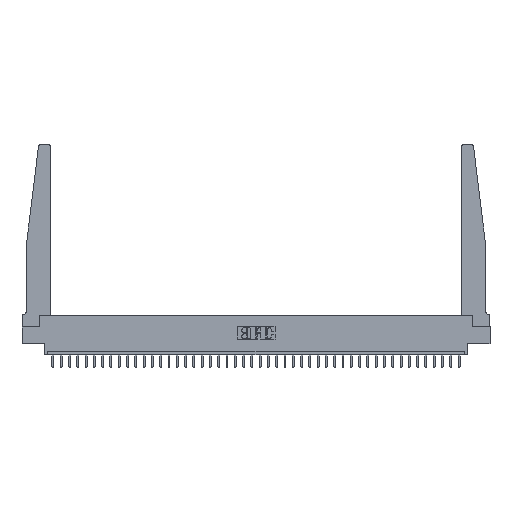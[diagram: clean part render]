
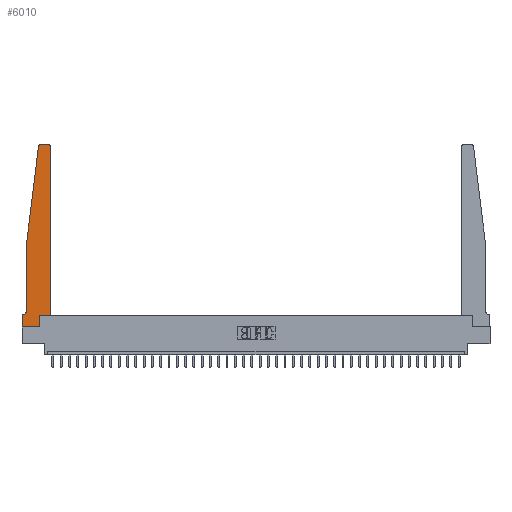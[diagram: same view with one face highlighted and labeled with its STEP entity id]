
A CAD part, top view. The second image highlights one B-rep face of the part: STEP entity #6010.
In plain terms, the highlighted planar face has unit normal (0, 0, 1).
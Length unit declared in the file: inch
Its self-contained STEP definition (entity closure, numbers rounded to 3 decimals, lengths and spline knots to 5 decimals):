
#558 = CARTESIAN_POINT ( 'NONE',  ( 0.065, 1.25, 0.37 ) ) ;
#587 = CARTESIAN_POINT ( 'NONE',  ( 0.065, 1.25, 0.37 ) ) ;
#779 = VECTOR ( 'NONE', #24021, 39.37008 ) ;
#856 = VERTEX_POINT ( 'NONE', #21070 ) ;
#1024 = VERTEX_POINT ( 'NONE', #10144 ) ;
#1655 = DIRECTION ( 'NONE',  ( 0., 1., 0. ) ) ;
#1832 = CARTESIAN_POINT ( 'NONE',  ( 0., 0.1875, 0.37 ) ) ;
#2166 = DIRECTION ( 'NONE',  ( 0., 0., -1. ) ) ;
#2306 = CARTESIAN_POINT ( 'NONE',  ( 0.27653, 2.72, 0.37 ) ) ;
#3428 = EDGE_CURVE ( 'NONE', #25080, #15302, #9215, .T. ) ;
#4819 = DIRECTION ( 'NONE',  ( 0., -1., 0. ) ) ;
#5062 = LINE ( 'NONE', #22486, #21195 ) ;
#5233 = VECTOR ( 'NONE', #21370, 39.37008 ) ;
#5399 = AXIS2_PLACEMENT_3D ( 'NONE', #24144, #2166, #29606 ) ;
#6010 = ADVANCED_FACE ( 'NONE', ( #11572 ), #15756, .T. ) ;
#6064 = EDGE_CURVE ( 'NONE', #11820, #20623, #17079, .T. ) ;
#6238 = LINE ( 'NONE', #587, #24451 ) ;
#6277 = EDGE_CURVE ( 'NONE', #20623, #12182, #6449, .T. ) ;
#6449 = CIRCLE ( 'NONE', #5399, 0.05 ) ;
#6466 = DIRECTION ( 'NONE',  ( 1., 0., 0. ) ) ;
#6562 = ORIENTED_EDGE ( 'NONE', *, *, #6064, .T. ) ;
#7493 = CARTESIAN_POINT ( 'NONE',  ( 0.425, 0.18, 0.37 ) ) ;
#9215 = LINE ( 'NONE', #16953, #24053 ) ;
#9612 = EDGE_CURVE ( 'NONE', #856, #20183, #13730, .T. ) ;
#9614 = CARTESIAN_POINT ( 'NONE',  ( 0.065, 0.1875, 0.37 ) ) ;
#9707 = LINE ( 'NONE', #13720, #34671 ) ;
#9741 = ORIENTED_EDGE ( 'NONE', *, *, #3428, .T. ) ;
#9880 = CARTESIAN_POINT ( 'NONE',  ( 0., 0., 0.37 ) ) ;
#10144 = CARTESIAN_POINT ( 'NONE',  ( 0., 0.1875, 0.37 ) ) ;
#10590 = AXIS2_PLACEMENT_3D ( 'NONE', #2306, #18377, #20989 ) ;
#11152 = LINE ( 'NONE', #9614, #17508 ) ;
#11572 = FACE_OUTER_BOUND ( 'NONE', #13483, .T. ) ;
#11820 = VERTEX_POINT ( 'NONE', #558 ) ;
#12182 = VERTEX_POINT ( 'NONE', #18285 ) ;
#12961 = CARTESIAN_POINT ( 'NONE',  ( 0.2605, 0.18, 0.37 ) ) ;
#13011 = EDGE_CURVE ( 'NONE', #1024, #16116, #9707, .T. ) ;
#13483 = EDGE_LOOP ( 'NONE', ( #28236, #22872, #15942, #6562, #14716, #17253, #27853, #21264, #21352, #15032, #9741, #23097 ) ) ;
#13720 = CARTESIAN_POINT ( 'NONE',  ( 0., 0., 0.37 ) ) ;
#13730 = LINE ( 'NONE', #12961, #5233 ) ;
#14716 = ORIENTED_EDGE ( 'NONE', *, *, #6277, .T. ) ;
#14963 = CARTESIAN_POINT ( 'NONE',  ( 0.27653, 2.75, 0.37 ) ) ;
#15032 = ORIENTED_EDGE ( 'NONE', *, *, #30413, .T. ) ;
#15148 = AXIS2_PLACEMENT_3D ( 'NONE', #1832, #18485, #32083 ) ;
#15302 = VERTEX_POINT ( 'NONE', #17391 ) ;
#15756 = PLANE ( 'NONE',  #15148 ) ;
#15942 = ORIENTED_EDGE ( 'NONE', *, *, #27890, .T. ) ;
#16116 = VERTEX_POINT ( 'NONE', #9880 ) ;
#16468 = DIRECTION ( 'NONE',  ( 0., -1., 0. ) ) ;
#16653 = EDGE_CURVE ( 'NONE', #24410, #29424, #30445, .T. ) ;
#16739 = AXIS2_PLACEMENT_3D ( 'NONE', #28509, #25639, #6466 ) ;
#16872 = DIRECTION ( 'NONE',  ( -0.122, -0.992, 0. ) ) ;
#16953 = CARTESIAN_POINT ( 'NONE',  ( 0.425, 0.18, 0.37 ) ) ;
#17079 = LINE ( 'NONE', #34515, #32295 ) ;
#17162 = CARTESIAN_POINT ( 'NONE',  ( 0.425, 0.18, 0.37 ) ) ;
#17253 = ORIENTED_EDGE ( 'NONE', *, *, #20396, .T. ) ;
#17391 = CARTESIAN_POINT ( 'NONE',  ( 0.425, 2.72, 0.37 ) ) ;
#17508 = VECTOR ( 'NONE', #18240, 39.37008 ) ;
#18240 = DIRECTION ( 'NONE',  ( -1., 0., 0. ) ) ;
#18285 = CARTESIAN_POINT ( 'NONE',  ( 0.015, 0.1875, 0.37 ) ) ;
#18377 = DIRECTION ( 'NONE',  ( 0., 0., 1. ) ) ;
#18485 = DIRECTION ( 'NONE',  ( 0., 0., 1. ) ) ;
#19468 = CARTESIAN_POINT ( 'NONE',  ( 0.2605, 0.18, 0.37 ) ) ;
#20010 = DIRECTION ( 'NONE',  ( -1., 0., 0. ) ) ;
#20183 = VERTEX_POINT ( 'NONE', #19468 ) ;
#20298 = CARTESIAN_POINT ( 'NONE',  ( 0.395, 2.75, 0.37 ) ) ;
#20396 = EDGE_CURVE ( 'NONE', #12182, #1024, #11152, .T. ) ;
#20623 = VERTEX_POINT ( 'NONE', #24862 ) ;
#20989 = DIRECTION ( 'NONE',  ( 1., 0., 0. ) ) ;
#21070 = CARTESIAN_POINT ( 'NONE',  ( 0.2605, 0., 0.37 ) ) ;
#21195 = VECTOR ( 'NONE', #20010, 39.37008 ) ;
#21264 = ORIENTED_EDGE ( 'NONE', *, *, #32529, .T. ) ;
#21352 = ORIENTED_EDGE ( 'NONE', *, *, #9612, .T. ) ;
#21370 = DIRECTION ( 'NONE',  ( 0., 1., 0. ) ) ;
#22380 = DIRECTION ( 'NONE',  ( 1., 0., 0. ) ) ;
#22486 = CARTESIAN_POINT ( 'NONE',  ( 0.25, 2.75, 0.37 ) ) ;
#22872 = ORIENTED_EDGE ( 'NONE', *, *, #16653, .T. ) ;
#23097 = ORIENTED_EDGE ( 'NONE', *, *, #28793, .T. ) ;
#24021 = DIRECTION ( 'NONE',  ( 1., 0., 0. ) ) ;
#24053 = VECTOR ( 'NONE', #1655, 39.37008 ) ;
#24144 = CARTESIAN_POINT ( 'NONE',  ( 0.015, 0.2375, 0.37 ) ) ;
#24410 = VERTEX_POINT ( 'NONE', #14963 ) ;
#24451 = VECTOR ( 'NONE', #16872, 39.37008 ) ;
#24862 = CARTESIAN_POINT ( 'NONE',  ( 0.065, 0.2375, 0.37 ) ) ;
#25080 = VERTEX_POINT ( 'NONE', #7493 ) ;
#25639 = DIRECTION ( 'NONE',  ( 0., 0., 1. ) ) ;
#26297 = EDGE_CURVE ( 'NONE', #33862, #24410, #5062, .T. ) ;
#26689 = LINE ( 'NONE', #17162, #30982 ) ;
#26847 = CARTESIAN_POINT ( 'NONE',  ( 0., 0., 0.37 ) ) ;
#27826 = LINE ( 'NONE', #26847, #779 ) ;
#27853 = ORIENTED_EDGE ( 'NONE', *, *, #13011, .T. ) ;
#27890 = EDGE_CURVE ( 'NONE', #29424, #11820, #6238, .T. ) ;
#28236 = ORIENTED_EDGE ( 'NONE', *, *, #26297, .T. ) ;
#28509 = CARTESIAN_POINT ( 'NONE',  ( 0.395, 2.72, 0.37 ) ) ;
#28793 = EDGE_CURVE ( 'NONE', #15302, #33862, #33271, .T. ) ;
#29424 = VERTEX_POINT ( 'NONE', #31453 ) ;
#29606 = DIRECTION ( 'NONE',  ( -1., 0., 0. ) ) ;
#30413 = EDGE_CURVE ( 'NONE', #20183, #25080, #26689, .T. ) ;
#30445 = CIRCLE ( 'NONE', #10590, 0.03 ) ;
#30982 = VECTOR ( 'NONE', #22380, 39.37008 ) ;
#31453 = CARTESIAN_POINT ( 'NONE',  ( 0.24675, 2.72367, 0.37 ) ) ;
#32083 = DIRECTION ( 'NONE',  ( 1., 0., 0. ) ) ;
#32295 = VECTOR ( 'NONE', #4819, 39.37008 ) ;
#32529 = EDGE_CURVE ( 'NONE', #16116, #856, #27826, .T. ) ;
#33271 = CIRCLE ( 'NONE', #16739, 0.03 ) ;
#33862 = VERTEX_POINT ( 'NONE', #20298 ) ;
#34515 = CARTESIAN_POINT ( 'NONE',  ( 0.065, 1.25, 0.37 ) ) ;
#34671 = VECTOR ( 'NONE', #16468, 39.37008 ) ;
